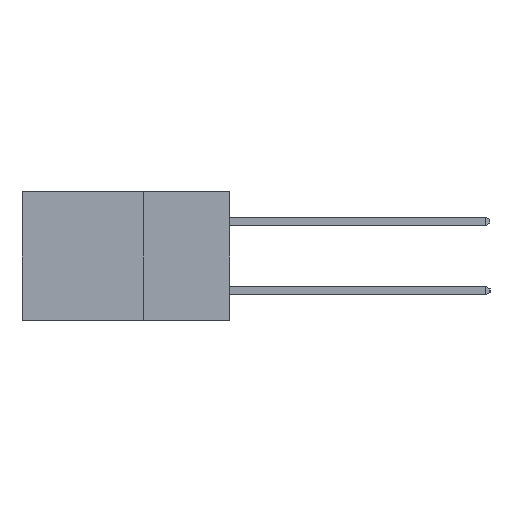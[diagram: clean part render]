
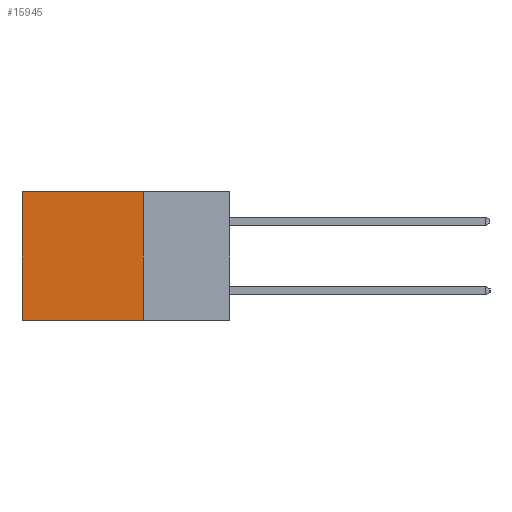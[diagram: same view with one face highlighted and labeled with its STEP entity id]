
A CAD part, left-side view. The second image highlights one B-rep face of the part: STEP entity #15945.
In plain terms, the highlighted planar face has unit normal (-1, 0, 0).
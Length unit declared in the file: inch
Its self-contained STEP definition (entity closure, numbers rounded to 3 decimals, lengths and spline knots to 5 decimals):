
#424 = CARTESIAN_POINT ( 'NONE',  ( 0.2615, 0.25, -0.37 ) ) ;
#701 = ORIENTED_EDGE ( 'NONE', *, *, #1158, .T. ) ;
#747 = DIRECTION ( 'NONE',  ( 0., 0., -1. ) ) ;
#1158 = EDGE_CURVE ( 'NONE', #3045, #10288, #6558, .T. ) ;
#2285 = FACE_OUTER_BOUND ( 'NONE', #16566, .T. ) ;
#2618 = CARTESIAN_POINT ( 'NONE',  ( 0.2615, 0.25, -0.37 ) ) ;
#2619 = VECTOR ( 'NONE', #7295, 39.37008 ) ;
#2700 = ORIENTED_EDGE ( 'NONE', *, *, #6840, .T. ) ;
#3007 = CARTESIAN_POINT ( 'NONE',  ( 0.2615, 0.6, -0.37 ) ) ;
#3045 = VERTEX_POINT ( 'NONE', #9650 ) ;
#4034 = AXIS2_PLACEMENT_3D ( 'NONE', #18628, #9768, #747 ) ;
#4516 = EDGE_CURVE ( 'NONE', #12478, #16106, #8558, .T. ) ;
#4973 = CARTESIAN_POINT ( 'NONE',  ( 0.2615, 0.25, 0. ) ) ;
#5110 = DIRECTION ( 'NONE',  ( 0., 0., -1. ) ) ;
#5265 = PLANE ( 'NONE',  #4034 ) ;
#5606 = VECTOR ( 'NONE', #5110, 39.37008 ) ;
#5736 = CARTESIAN_POINT ( 'NONE',  ( 0.2615, 0.25, -0.37 ) ) ;
#5791 = CARTESIAN_POINT ( 'NONE',  ( 0.2615, 0.25, 0. ) ) ;
#6558 = LINE ( 'NONE', #3007, #5606 ) ;
#6617 = LINE ( 'NONE', #5791, #2619 ) ;
#6840 = EDGE_CURVE ( 'NONE', #12478, #3045, #6617, .T. ) ;
#7295 = DIRECTION ( 'NONE',  ( 0., 1., 0. ) ) ;
#8097 = VECTOR ( 'NONE', #17607, 39.37008 ) ;
#8404 = EDGE_CURVE ( 'NONE', #16106, #10288, #10298, .T. ) ;
#8405 = ORIENTED_EDGE ( 'NONE', *, *, #4516, .F. ) ;
#8558 = LINE ( 'NONE', #5736, #8097 ) ;
#9650 = CARTESIAN_POINT ( 'NONE',  ( 0.2615, 0.6, 0. ) ) ;
#9768 = DIRECTION ( 'NONE',  ( 1., 0., 0. ) ) ;
#10288 = VERTEX_POINT ( 'NONE', #15832 ) ;
#10298 = LINE ( 'NONE', #424, #14682 ) ;
#10974 = DIRECTION ( 'NONE',  ( 0., 1., 0. ) ) ;
#12478 = VERTEX_POINT ( 'NONE', #4973 ) ;
#14682 = VECTOR ( 'NONE', #10974, 39.37008 ) ;
#15832 = CARTESIAN_POINT ( 'NONE',  ( 0.2615, 0.6, -0.37 ) ) ;
#15945 = ADVANCED_FACE ( 'NONE', ( #2285 ), #5265, .F. ) ;
#15986 = ORIENTED_EDGE ( 'NONE', *, *, #8404, .F. ) ;
#16106 = VERTEX_POINT ( 'NONE', #2618 ) ;
#16566 = EDGE_LOOP ( 'NONE', ( #701, #15986, #8405, #2700 ) ) ;
#17607 = DIRECTION ( 'NONE',  ( 0., 0., -1. ) ) ;
#18628 = CARTESIAN_POINT ( 'NONE',  ( 0.2615, 0.25, -0.37 ) ) ;
